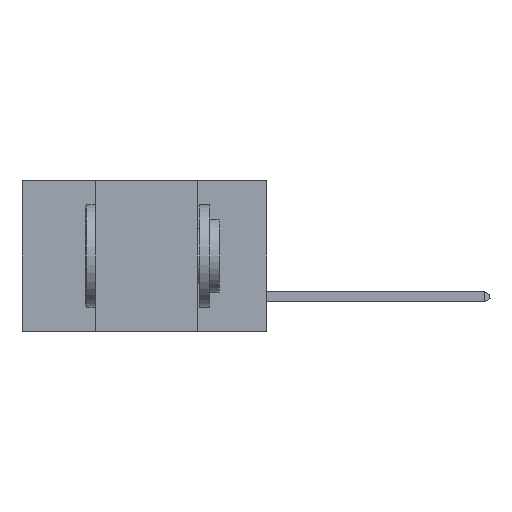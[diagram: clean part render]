
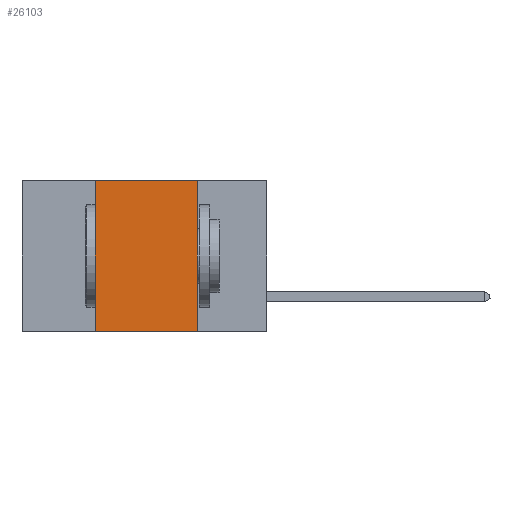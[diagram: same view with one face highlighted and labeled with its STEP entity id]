
A CAD part, left-side view. The second image highlights one B-rep face of the part: STEP entity #26103.
In plain terms, the highlighted planar face has unit normal (-1, 0, 0).
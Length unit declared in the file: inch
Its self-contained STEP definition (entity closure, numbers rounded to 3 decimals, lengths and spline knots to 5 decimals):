
#148 = EDGE_CURVE ( 'NONE', #20099, #8895, #3238, .T. ) ;
#1508 = ORIENTED_EDGE ( 'NONE', *, *, #24588, .F. ) ;
#2605 = CARTESIAN_POINT ( 'NONE',  ( 0., 0.6, -0.37 ) ) ;
#3238 = LINE ( 'NONE', #2605, #17360 ) ;
#4586 = CARTESIAN_POINT ( 'NONE',  ( 0., 0.17, 0. ) ) ;
#4835 = FACE_OUTER_BOUND ( 'NONE', #14654, .T. ) ;
#7493 = CARTESIAN_POINT ( 'NONE',  ( 0., 0.17, 0. ) ) ;
#8668 = EDGE_CURVE ( 'NONE', #21123, #21549, #22466, .T. ) ;
#8895 = VERTEX_POINT ( 'NONE', #24753 ) ;
#9237 = ORIENTED_EDGE ( 'NONE', *, *, #13618, .F. ) ;
#9529 = DIRECTION ( 'NONE',  ( 0., 0., -1. ) ) ;
#10248 = CARTESIAN_POINT ( 'NONE',  ( 0., 0.6, 0. ) ) ;
#11584 = VECTOR ( 'NONE', #27075, 39.37008 ) ;
#12826 = PLANE ( 'NONE',  #19925 ) ;
#13618 = EDGE_CURVE ( 'NONE', #20099, #21123, #19042, .T. ) ;
#14654 = EDGE_LOOP ( 'NONE', ( #1508, #18312, #9237, #20215 ) ) ;
#15681 = CARTESIAN_POINT ( 'NONE',  ( 0., 0.6, 0. ) ) ;
#16206 = CARTESIAN_POINT ( 'NONE',  ( 0., 0.42, 0. ) ) ;
#17322 = LINE ( 'NONE', #4586, #21592 ) ;
#17359 = DIRECTION ( 'NONE',  ( 1., 0., 0. ) ) ;
#17360 = VECTOR ( 'NONE', #18448, 39.37008 ) ;
#17980 = DIRECTION ( 'NONE',  ( 0., -1., 0. ) ) ;
#18312 = ORIENTED_EDGE ( 'NONE', *, *, #8668, .F. ) ;
#18448 = DIRECTION ( 'NONE',  ( 0., -1., 0. ) ) ;
#19042 = LINE ( 'NONE', #29274, #11584 ) ;
#19925 = AXIS2_PLACEMENT_3D ( 'NONE', #10248, #17359, #28652 ) ;
#20099 = VERTEX_POINT ( 'NONE', #24196 ) ;
#20215 = ORIENTED_EDGE ( 'NONE', *, *, #148, .T. ) ;
#21123 = VERTEX_POINT ( 'NONE', #16206 ) ;
#21430 = VECTOR ( 'NONE', #17980, 39.37008 ) ;
#21549 = VERTEX_POINT ( 'NONE', #7493 ) ;
#21592 = VECTOR ( 'NONE', #9529, 39.37008 ) ;
#22466 = LINE ( 'NONE', #15681, #21430 ) ;
#24196 = CARTESIAN_POINT ( 'NONE',  ( 0., 0.42, -0.37 ) ) ;
#24588 = EDGE_CURVE ( 'NONE', #21549, #8895, #17322, .T. ) ;
#24753 = CARTESIAN_POINT ( 'NONE',  ( 0., 0.17, -0.37 ) ) ;
#26103 = ADVANCED_FACE ( 'NONE', ( #4835 ), #12826, .F. ) ;
#27075 = DIRECTION ( 'NONE',  ( 0., 0., 1. ) ) ;
#28652 = DIRECTION ( 'NONE',  ( 0., 0., -1. ) ) ;
#29274 = CARTESIAN_POINT ( 'NONE',  ( 0., 0.42, 0. ) ) ;
